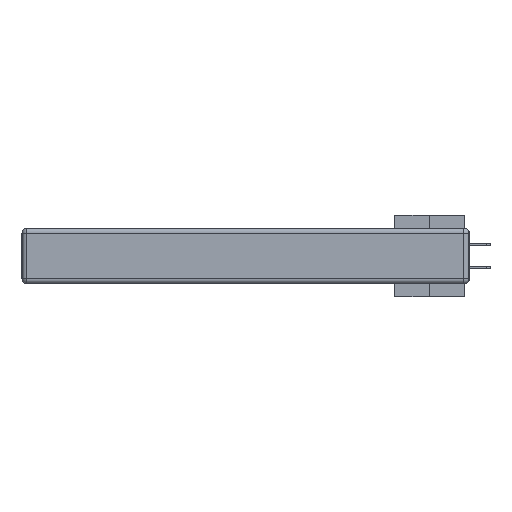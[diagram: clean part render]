
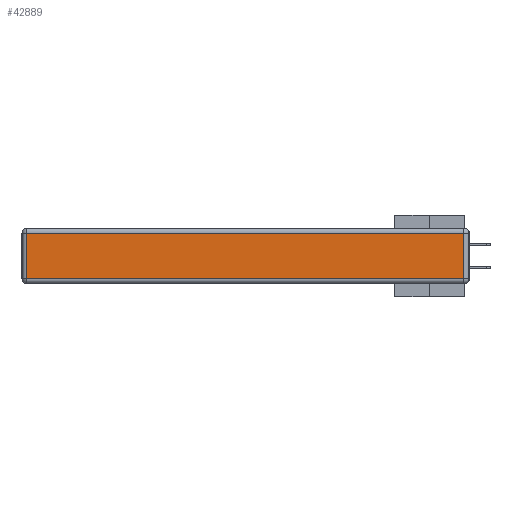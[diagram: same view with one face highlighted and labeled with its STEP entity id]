
A CAD part, left-side view. The second image highlights one B-rep face of the part: STEP entity #42889.
In plain terms, the highlighted planar face has unit normal (-1, 0, 0).
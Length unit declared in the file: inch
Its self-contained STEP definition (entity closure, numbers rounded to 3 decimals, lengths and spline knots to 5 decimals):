
#14 = LINE ( 'NONE', #44665, #1163 ) ;
#362 = CARTESIAN_POINT ( 'NONE',  ( 0., 2.72, -0.03 ) ) ;
#669 = CARTESIAN_POINT ( 'NONE',  ( 0., 2.72, -0.313 ) ) ;
#1163 = VECTOR ( 'NONE', #37355, 39.37008 ) ;
#1438 = VERTEX_POINT ( 'NONE', #362 ) ;
#3791 = EDGE_CURVE ( 'NONE', #1438, #45560, #14, .T. ) ;
#4461 = DIRECTION ( 'NONE',  ( 0., 0., 1. ) ) ;
#4683 = VERTEX_POINT ( 'NONE', #7972 ) ;
#6854 = EDGE_CURVE ( 'NONE', #45560, #9825, #36080, .T. ) ;
#7972 = CARTESIAN_POINT ( 'NONE',  ( 0., 0.03, -0.03 ) ) ;
#9825 = VERTEX_POINT ( 'NONE', #18454 ) ;
#11013 = DIRECTION ( 'NONE',  ( 0., 1., 0. ) ) ;
#11931 = PLANE ( 'NONE',  #13765 ) ;
#13765 = AXIS2_PLACEMENT_3D ( 'NONE', #26109, #18660, #4461 ) ;
#14283 = DIRECTION ( 'NONE',  ( 0., -1., 0. ) ) ;
#14922 = LINE ( 'NONE', #36434, #29479 ) ;
#16129 = ORIENTED_EDGE ( 'NONE', *, *, #16834, .T. ) ;
#16834 = EDGE_CURVE ( 'NONE', #9825, #4683, #25639, .T. ) ;
#17990 = ORIENTED_EDGE ( 'NONE', *, *, #3791, .T. ) ;
#18454 = CARTESIAN_POINT ( 'NONE',  ( 0., 0.03, -0.313 ) ) ;
#18660 = DIRECTION ( 'NONE',  ( -1., 0., 0. ) ) ;
#18754 = DIRECTION ( 'NONE',  ( 0., 0., 1. ) ) ;
#19718 = ORIENTED_EDGE ( 'NONE', *, *, #23332, .T. ) ;
#23332 = EDGE_CURVE ( 'NONE', #4683, #1438, #14922, .T. ) ;
#25639 = LINE ( 'NONE', #40234, #40118 ) ;
#26109 = CARTESIAN_POINT ( 'NONE',  ( 0., 0., -0.343 ) ) ;
#26450 = EDGE_LOOP ( 'NONE', ( #32993, #16129, #19718, #17990 ) ) ;
#26569 = VECTOR ( 'NONE', #14283, 39.37008 ) ;
#29479 = VECTOR ( 'NONE', #11013, 39.37008 ) ;
#32251 = CARTESIAN_POINT ( 'NONE',  ( 0., 0., -0.313 ) ) ;
#32993 = ORIENTED_EDGE ( 'NONE', *, *, #6854, .T. ) ;
#36080 = LINE ( 'NONE', #32251, #26569 ) ;
#36434 = CARTESIAN_POINT ( 'NONE',  ( 0., 2.75, -0.03 ) ) ;
#37355 = DIRECTION ( 'NONE',  ( 0., 0., -1. ) ) ;
#40118 = VECTOR ( 'NONE', #18754, 39.37008 ) ;
#40234 = CARTESIAN_POINT ( 'NONE',  ( 0., 0.03, -0.343 ) ) ;
#41834 = FACE_OUTER_BOUND ( 'NONE', #26450, .T. ) ;
#42889 = ADVANCED_FACE ( 'NONE', ( #41834 ), #11931, .T. ) ;
#44665 = CARTESIAN_POINT ( 'NONE',  ( 0., 2.72, -0.343 ) ) ;
#45560 = VERTEX_POINT ( 'NONE', #669 ) ;
